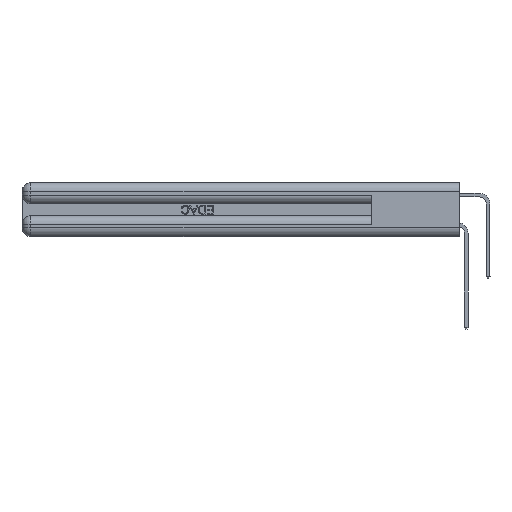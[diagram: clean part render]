
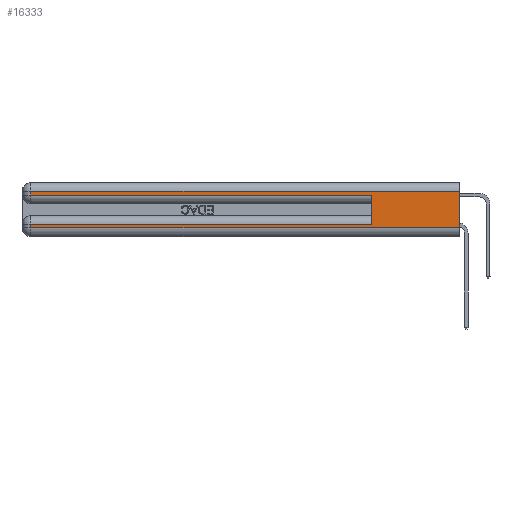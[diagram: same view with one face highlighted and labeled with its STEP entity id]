
A CAD part, left-side view. The second image highlights one B-rep face of the part: STEP entity #16333.
In plain terms, the highlighted planar face has unit normal (-1, 0, 0).
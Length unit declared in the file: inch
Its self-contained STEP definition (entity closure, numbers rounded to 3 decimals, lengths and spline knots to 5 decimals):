
#1307 = EDGE_LOOP ( 'NONE', ( #43138, #26651, #37159, #2885, #12371, #31093, #41533, #14597 ) ) ;
#1388 = DIRECTION ( 'NONE',  ( 0., 1., 0. ) ) ;
#2885 = ORIENTED_EDGE ( 'NONE', *, *, #24427, .T. ) ;
#3561 = CARTESIAN_POINT ( 'NONE',  ( 0., 0., 0.06 ) ) ;
#3674 = EDGE_CURVE ( 'NONE', #9455, #13243, #42626, .T. ) ;
#3935 = EDGE_CURVE ( 'NONE', #22102, #5163, #22268, .T. ) ;
#5163 = VERTEX_POINT ( 'NONE', #28912 ) ;
#6999 = LINE ( 'NONE', #16859, #25775 ) ;
#9455 = VERTEX_POINT ( 'NONE', #43190 ) ;
#10249 = EDGE_CURVE ( 'NONE', #11243, #26199, #27776, .T. ) ;
#11243 = VERTEX_POINT ( 'NONE', #42072 ) ;
#11552 = DIRECTION ( 'NONE',  ( 0., 0., -1. ) ) ;
#11722 = CARTESIAN_POINT ( 'NONE',  ( 0., 2.94, 0.285 ) ) ;
#11999 = VERTEX_POINT ( 'NONE', #11722 ) ;
#12371 = ORIENTED_EDGE ( 'NONE', *, *, #10249, .F. ) ;
#12608 = PLANE ( 'NONE',  #39580 ) ;
#12686 = LINE ( 'NONE', #36778, #20929 ) ;
#13059 = VERTEX_POINT ( 'NONE', #35458 ) ;
#13243 = VERTEX_POINT ( 'NONE', #29427 ) ;
#14597 = ORIENTED_EDGE ( 'NONE', *, *, #38005, .T. ) ;
#15767 = CARTESIAN_POINT ( 'NONE',  ( 0., 0., 0.085 ) ) ;
#16168 = DIRECTION ( 'NONE',  ( 1., 0., 0. ) ) ;
#16333 = ADVANCED_FACE ( 'NONE', ( #34841 ), #12608, .F. ) ;
#16859 = CARTESIAN_POINT ( 'NONE',  ( 0., 0., 0.285 ) ) ;
#19071 = CARTESIAN_POINT ( 'NONE',  ( 0., 0., 0.31 ) ) ;
#19210 = DIRECTION ( 'NONE',  ( 0., 0., -1. ) ) ;
#19285 = DIRECTION ( 'NONE',  ( 0., 1., 0. ) ) ;
#20929 = VECTOR ( 'NONE', #19210, 39.37008 ) ;
#22069 = VECTOR ( 'NONE', #19285, 39.37008 ) ;
#22102 = VERTEX_POINT ( 'NONE', #22249 ) ;
#22249 = CARTESIAN_POINT ( 'NONE',  ( 0., 2.94, 0.085 ) ) ;
#22268 = LINE ( 'NONE', #29186, #39899 ) ;
#22927 = EDGE_CURVE ( 'NONE', #11243, #22102, #32556, .T. ) ;
#23034 = CARTESIAN_POINT ( 'NONE',  ( 0., 0., 0.37 ) ) ;
#23527 = EDGE_CURVE ( 'NONE', #9455, #13059, #25856, .T. ) ;
#24427 = EDGE_CURVE ( 'NONE', #11999, #26199, #6999, .T. ) ;
#25775 = VECTOR ( 'NONE', #41441, 39.37008 ) ;
#25856 = LINE ( 'NONE', #19071, #43457 ) ;
#26199 = VERTEX_POINT ( 'NONE', #40430 ) ;
#26319 = DIRECTION ( 'NONE',  ( 0., 0., 1. ) ) ;
#26651 = ORIENTED_EDGE ( 'NONE', *, *, #23527, .T. ) ;
#26654 = VECTOR ( 'NONE', #26319, 39.37008 ) ;
#27776 = LINE ( 'NONE', #40326, #26654 ) ;
#28312 = DIRECTION ( 'NONE',  ( 0., -1., 0. ) ) ;
#28912 = CARTESIAN_POINT ( 'NONE',  ( 0., 2.94, 0.06 ) ) ;
#29186 = CARTESIAN_POINT ( 'NONE',  ( 0., 2.94, 0.37 ) ) ;
#29427 = CARTESIAN_POINT ( 'NONE',  ( 0., 0., 0.06 ) ) ;
#29834 = LINE ( 'NONE', #3561, #38095 ) ;
#31093 = ORIENTED_EDGE ( 'NONE', *, *, #22927, .T. ) ;
#32556 = LINE ( 'NONE', #15767, #22069 ) ;
#33336 = VECTOR ( 'NONE', #11552, 39.37008 ) ;
#34841 = FACE_OUTER_BOUND ( 'NONE', #1307, .T. ) ;
#35458 = CARTESIAN_POINT ( 'NONE',  ( 0., 2.94, 0.31 ) ) ;
#36290 = DIRECTION ( 'NONE',  ( 0., 0., -1. ) ) ;
#36778 = CARTESIAN_POINT ( 'NONE',  ( 0., 2.94, 0.37 ) ) ;
#37159 = ORIENTED_EDGE ( 'NONE', *, *, #40941, .T. ) ;
#38005 = EDGE_CURVE ( 'NONE', #5163, #13243, #29834, .T. ) ;
#38095 = VECTOR ( 'NONE', #28312, 39.37008 ) ;
#39580 = AXIS2_PLACEMENT_3D ( 'NONE', #23034, #16168, #40748 ) ;
#39899 = VECTOR ( 'NONE', #36290, 39.37008 ) ;
#40326 = CARTESIAN_POINT ( 'NONE',  ( 0., 0.6, 0.145 ) ) ;
#40430 = CARTESIAN_POINT ( 'NONE',  ( 0., 0.6, 0.285 ) ) ;
#40748 = DIRECTION ( 'NONE',  ( 0., 0., -1. ) ) ;
#40941 = EDGE_CURVE ( 'NONE', #13059, #11999, #12686, .T. ) ;
#41441 = DIRECTION ( 'NONE',  ( 0., -1., 0. ) ) ;
#41533 = ORIENTED_EDGE ( 'NONE', *, *, #3935, .T. ) ;
#42072 = CARTESIAN_POINT ( 'NONE',  ( 0., 0.6, 0.085 ) ) ;
#42626 = LINE ( 'NONE', #43212, #33336 ) ;
#43138 = ORIENTED_EDGE ( 'NONE', *, *, #3674, .F. ) ;
#43190 = CARTESIAN_POINT ( 'NONE',  ( 0., 0., 0.31 ) ) ;
#43212 = CARTESIAN_POINT ( 'NONE',  ( 0., 0., 0.37 ) ) ;
#43457 = VECTOR ( 'NONE', #1388, 39.37008 ) ;
